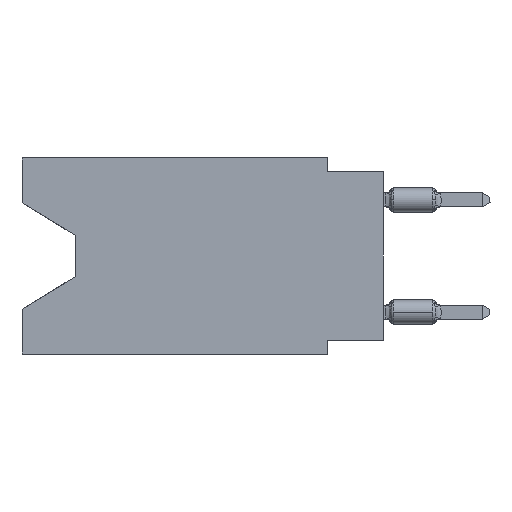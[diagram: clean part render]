
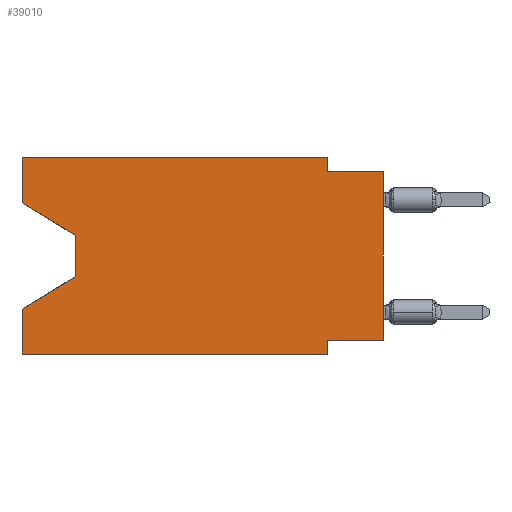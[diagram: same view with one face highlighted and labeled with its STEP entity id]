
A CAD part, left-side view. The second image highlights one B-rep face of the part: STEP entity #39010.
In plain terms, the highlighted planar face has unit normal (-1, 0, 0).
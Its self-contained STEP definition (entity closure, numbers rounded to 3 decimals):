
#275 = LINE ( 'NONE', #22624, #1048 ) ;
#590 = CARTESIAN_POINT ( 'NONE',  ( 0., 2.54, -8.89 ) ) ;
#603 = VECTOR ( 'NONE', #35610, 1000. ) ;
#765 = CARTESIAN_POINT ( 'NONE',  ( 0., 0., -0.635 ) ) ;
#886 = DIRECTION ( 'NONE',  ( 0., 0., -1. ) ) ;
#1048 = VECTOR ( 'NONE', #18047, 1000. ) ;
#2771 = CARTESIAN_POINT ( 'NONE',  ( 0., 2.54, -8.89 ) ) ;
#2801 = EDGE_CURVE ( 'NONE', #29773, #7335, #27170, .T. ) ;
#3575 = VECTOR ( 'NONE', #25034, 1000. ) ;
#4357 = VERTEX_POINT ( 'NONE', #14640 ) ;
#4568 = ORIENTED_EDGE ( 'NONE', *, *, #40398, .F. ) ;
#4777 = VECTOR ( 'NONE', #39951, 1000. ) ;
#5163 = LINE ( 'NONE', #590, #45197 ) ;
#5918 = CARTESIAN_POINT ( 'NONE',  ( 0., 2.54, 0. ) ) ;
#6010 = CARTESIAN_POINT ( 'NONE',  ( 0., 0., 0. ) ) ;
#6460 = VERTEX_POINT ( 'NONE', #2771 ) ;
#7335 = VERTEX_POINT ( 'NONE', #51020 ) ;
#7605 = VERTEX_POINT ( 'NONE', #48437 ) ;
#7677 = CARTESIAN_POINT ( 'NONE',  ( 0., 13.97, -5.385 ) ) ;
#7791 = VERTEX_POINT ( 'NONE', #52018 ) ;
#9886 = VECTOR ( 'NONE', #50319, 1000. ) ;
#10551 = ORIENTED_EDGE ( 'NONE', *, *, #25519, .F. ) ;
#10580 = LINE ( 'NONE', #27521, #11800 ) ;
#10807 = VECTOR ( 'NONE', #33307, 1000. ) ;
#10819 = ORIENTED_EDGE ( 'NONE', *, *, #28760, .T. ) ;
#11072 = LINE ( 'NONE', #42019, #9886 ) ;
#11135 = DIRECTION ( 'NONE',  ( 0., 0.855, -0.519 ) ) ;
#11800 = VECTOR ( 'NONE', #11135, 1000. ) ;
#11815 = EDGE_LOOP ( 'NONE', ( #13872, #10819, #48685, #49385, #48019, #28874, #4568, #35143, #19844, #45615, #10551, #14434 ) ) ;
#11858 = LINE ( 'NONE', #12715, #603 ) ;
#12715 = CARTESIAN_POINT ( 'NONE',  ( 0., 13.97, -3.505 ) ) ;
#13872 = ORIENTED_EDGE ( 'NONE', *, *, #55470, .T. ) ;
#14434 = ORIENTED_EDGE ( 'NONE', *, *, #21472, .F. ) ;
#14548 = VECTOR ( 'NONE', #41728, 1000. ) ;
#14640 = CARTESIAN_POINT ( 'NONE',  ( 0., 16.383, 0. ) ) ;
#15970 = VECTOR ( 'NONE', #53004, 1000. ) ;
#16451 = LINE ( 'NONE', #47349, #3575 ) ;
#18047 = DIRECTION ( 'NONE',  ( 0., -1., 0. ) ) ;
#19242 = LINE ( 'NONE', #53303, #27126 ) ;
#19844 = ORIENTED_EDGE ( 'NONE', *, *, #52382, .F. ) ;
#19868 = VERTEX_POINT ( 'NONE', #765 ) ;
#21472 = EDGE_CURVE ( 'NONE', #46656, #4357, #19242, .T. ) ;
#22482 = LINE ( 'NONE', #52823, #4777 ) ;
#22624 = CARTESIAN_POINT ( 'NONE',  ( 0., 16.383, -8.89 ) ) ;
#23023 = AXIS2_PLACEMENT_3D ( 'NONE', #46369, #42343, #38040 ) ;
#24867 = EDGE_CURVE ( 'NONE', #54093, #7335, #10580, .T. ) ;
#25034 = DIRECTION ( 'NONE',  ( 0., -1., 0. ) ) ;
#25235 = CARTESIAN_POINT ( 'NONE',  ( 0., 0., -0.635 ) ) ;
#25519 = EDGE_CURVE ( 'NONE', #4357, #54310, #16451, .T. ) ;
#27126 = VECTOR ( 'NONE', #49873, 1000. ) ;
#27170 = LINE ( 'NONE', #28843, #14548 ) ;
#27521 = CARTESIAN_POINT ( 'NONE',  ( 0., 13.97, -5.385 ) ) ;
#28181 = CARTESIAN_POINT ( 'NONE',  ( 0., 2.54, 0. ) ) ;
#28480 = VECTOR ( 'NONE', #42688, 1000. ) ;
#28504 = CARTESIAN_POINT ( 'NONE',  ( 0., 2.54, -8.255 ) ) ;
#28760 = EDGE_CURVE ( 'NONE', #7605, #54093, #11858, .T. ) ;
#28843 = CARTESIAN_POINT ( 'NONE',  ( 0., 16.383, 0. ) ) ;
#28874 = ORIENTED_EDGE ( 'NONE', *, *, #32125, .F. ) ;
#29773 = VERTEX_POINT ( 'NONE', #56397 ) ;
#31601 = VERTEX_POINT ( 'NONE', #28504 ) ;
#32103 = EDGE_CURVE ( 'NONE', #7791, #19868, #32361, .T. ) ;
#32125 = EDGE_CURVE ( 'NONE', #31601, #6460, #5163, .T. ) ;
#32361 = LINE ( 'NONE', #6010, #15970 ) ;
#32737 = LINE ( 'NONE', #28181, #10807 ) ;
#33307 = DIRECTION ( 'NONE',  ( 0., 0., -1. ) ) ;
#33468 = FACE_OUTER_BOUND ( 'NONE', #11815, .T. ) ;
#35143 = ORIENTED_EDGE ( 'NONE', *, *, #32103, .T. ) ;
#35610 = DIRECTION ( 'NONE',  ( 0., 0., -1. ) ) ;
#38040 = DIRECTION ( 'NONE',  ( 0., 0., -1. ) ) ;
#39010 = ADVANCED_FACE ( 'NONE', ( #33468 ), #47203, .F. ) ;
#39951 = DIRECTION ( 'NONE',  ( 0., 1., 0. ) ) ;
#40398 = EDGE_CURVE ( 'NONE', #7791, #31601, #22482, .T. ) ;
#40530 = CARTESIAN_POINT ( 'NONE',  ( 0., 16.383, -2.038 ) ) ;
#41728 = DIRECTION ( 'NONE',  ( 0., 0., 1. ) ) ;
#42019 = CARTESIAN_POINT ( 'NONE',  ( 0., 16.383, -2.038 ) ) ;
#42343 = DIRECTION ( 'NONE',  ( 1., 0., 0. ) ) ;
#42403 = LINE ( 'NONE', #25235, #28480 ) ;
#42688 = DIRECTION ( 'NONE',  ( 0., -1., 0. ) ) ;
#45197 = VECTOR ( 'NONE', #886, 1000. ) ;
#45615 = ORIENTED_EDGE ( 'NONE', *, *, #55781, .F. ) ;
#46369 = CARTESIAN_POINT ( 'NONE',  ( 0., 16.383, 0. ) ) ;
#46656 = VERTEX_POINT ( 'NONE', #40530 ) ;
#47203 = PLANE ( 'NONE',  #23023 ) ;
#47349 = CARTESIAN_POINT ( 'NONE',  ( 0., 16.383, 0. ) ) ;
#48019 = ORIENTED_EDGE ( 'NONE', *, *, #52432, .T. ) ;
#48437 = CARTESIAN_POINT ( 'NONE',  ( 0., 13.97, -3.505 ) ) ;
#48685 = ORIENTED_EDGE ( 'NONE', *, *, #24867, .T. ) ;
#49385 = ORIENTED_EDGE ( 'NONE', *, *, #2801, .F. ) ;
#49873 = DIRECTION ( 'NONE',  ( 0., 0., 1. ) ) ;
#50319 = DIRECTION ( 'NONE',  ( 0., -0.855, -0.519 ) ) ;
#51020 = CARTESIAN_POINT ( 'NONE',  ( 0., 16.383, -6.852 ) ) ;
#51979 = CARTESIAN_POINT ( 'NONE',  ( 0., 2.54, -0.635 ) ) ;
#52018 = CARTESIAN_POINT ( 'NONE',  ( 0., 0., -8.255 ) ) ;
#52382 = EDGE_CURVE ( 'NONE', #52677, #19868, #42403, .T. ) ;
#52432 = EDGE_CURVE ( 'NONE', #29773, #6460, #275, .T. ) ;
#52677 = VERTEX_POINT ( 'NONE', #51979 ) ;
#52823 = CARTESIAN_POINT ( 'NONE',  ( 0., 0., -8.255 ) ) ;
#53004 = DIRECTION ( 'NONE',  ( 0., 0., 1. ) ) ;
#53303 = CARTESIAN_POINT ( 'NONE',  ( 0., 16.383, 0. ) ) ;
#54093 = VERTEX_POINT ( 'NONE', #7677 ) ;
#54310 = VERTEX_POINT ( 'NONE', #5918 ) ;
#55470 = EDGE_CURVE ( 'NONE', #46656, #7605, #11072, .T. ) ;
#55781 = EDGE_CURVE ( 'NONE', #54310, #52677, #32737, .T. ) ;
#56397 = CARTESIAN_POINT ( 'NONE',  ( 0., 16.383, -8.89 ) ) ;
